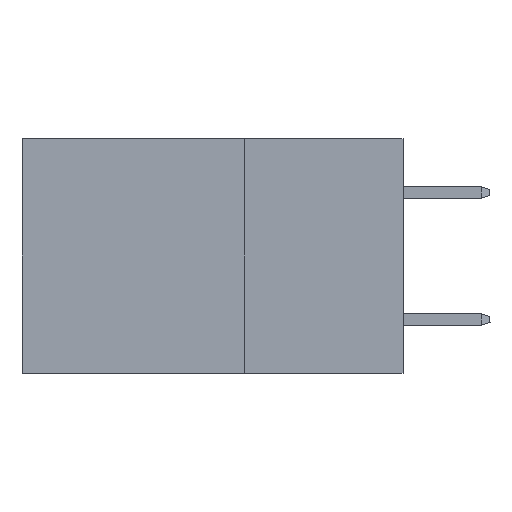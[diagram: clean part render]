
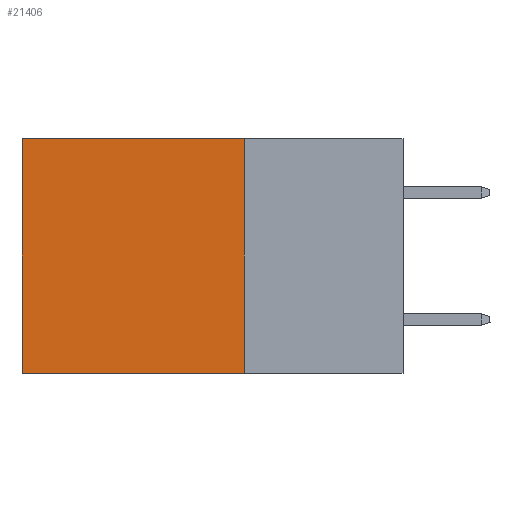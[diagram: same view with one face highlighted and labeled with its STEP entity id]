
A CAD part, left-side view. The second image highlights one B-rep face of the part: STEP entity #21406.
In plain terms, the highlighted planar face has unit normal (-1, 0, 0).
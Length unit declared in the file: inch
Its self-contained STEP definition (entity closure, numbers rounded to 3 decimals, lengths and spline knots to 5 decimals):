
#617 = CARTESIAN_POINT ( 'NONE',  ( 0.2875, 0.25, 0. ) ) ;
#1803 = VECTOR ( 'NONE', #14037, 39.37008 ) ;
#2261 = VECTOR ( 'NONE', #2532, 39.37008 ) ;
#2265 = LINE ( 'NONE', #10813, #2261 ) ;
#2532 = DIRECTION ( 'NONE',  ( 0., 1., 0. ) ) ;
#2801 = CARTESIAN_POINT ( 'NONE',  ( 0.2875, 0.25, 0. ) ) ;
#2837 = PLANE ( 'NONE',  #6535 ) ;
#3733 = ORIENTED_EDGE ( 'NONE', *, *, #25730, .F. ) ;
#4112 = ORIENTED_EDGE ( 'NONE', *, *, #26045, .F. ) ;
#6535 = AXIS2_PLACEMENT_3D ( 'NONE', #617, #7078, #21560 ) ;
#7078 = DIRECTION ( 'NONE',  ( 1., 0., 0. ) ) ;
#7593 = LINE ( 'NONE', #2801, #1803 ) ;
#7768 = EDGE_LOOP ( 'NONE', ( #8494, #3733, #4112, #12829 ) ) ;
#8494 = ORIENTED_EDGE ( 'NONE', *, *, #14402, .T. ) ;
#8809 = CARTESIAN_POINT ( 'NONE',  ( 0.2875, 0.25, 0. ) ) ;
#9035 = FACE_OUTER_BOUND ( 'NONE', #7768, .T. ) ;
#10813 = CARTESIAN_POINT ( 'NONE',  ( 0.2875, 0.25, 0. ) ) ;
#12829 = ORIENTED_EDGE ( 'NONE', *, *, #26012, .T. ) ;
#14037 = DIRECTION ( 'NONE',  ( 0., 0., -1. ) ) ;
#14402 = EDGE_CURVE ( 'NONE', #18473, #25778, #14671, .T. ) ;
#14671 = LINE ( 'NONE', #25334, #26999 ) ;
#18473 = VERTEX_POINT ( 'NONE', #27229 ) ;
#18846 = CARTESIAN_POINT ( 'NONE',  ( 0.2875, 0.25, -0.37 ) ) ;
#18957 = CARTESIAN_POINT ( 'NONE',  ( 0.2875, 0.6, -0.37 ) ) ;
#19279 = VERTEX_POINT ( 'NONE', #8809 ) ;
#19724 = VECTOR ( 'NONE', #27273, 39.37008 ) ;
#20798 = CARTESIAN_POINT ( 'NONE',  ( 0.2875, 0.25, -0.37 ) ) ;
#21406 = ADVANCED_FACE ( 'NONE', ( #9035 ), #2837, .F. ) ;
#21560 = DIRECTION ( 'NONE',  ( 0., 0., -1. ) ) ;
#21681 = VERTEX_POINT ( 'NONE', #18846 ) ;
#23341 = LINE ( 'NONE', #20798, #19724 ) ;
#25334 = CARTESIAN_POINT ( 'NONE',  ( 0.2875, 0.6, 0. ) ) ;
#25497 = DIRECTION ( 'NONE',  ( 0., 0., -1. ) ) ;
#25730 = EDGE_CURVE ( 'NONE', #21681, #25778, #23341, .T. ) ;
#25778 = VERTEX_POINT ( 'NONE', #18957 ) ;
#26012 = EDGE_CURVE ( 'NONE', #19279, #18473, #2265, .T. ) ;
#26045 = EDGE_CURVE ( 'NONE', #19279, #21681, #7593, .T. ) ;
#26999 = VECTOR ( 'NONE', #25497, 39.37008 ) ;
#27229 = CARTESIAN_POINT ( 'NONE',  ( 0.2875, 0.6, 0. ) ) ;
#27273 = DIRECTION ( 'NONE',  ( 0., 1., 0. ) ) ;
